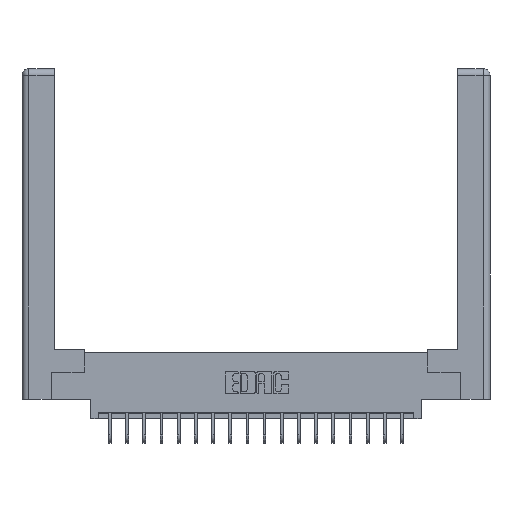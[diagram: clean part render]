
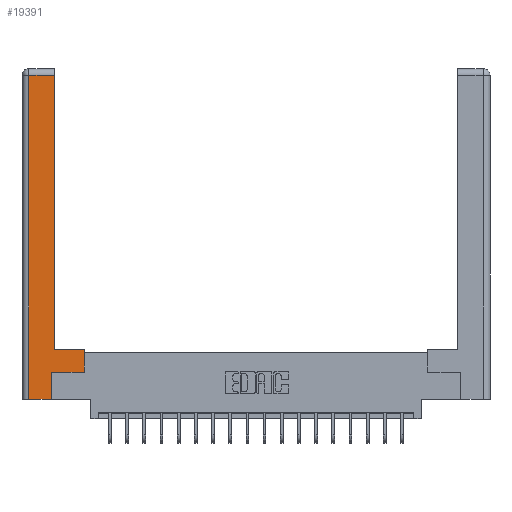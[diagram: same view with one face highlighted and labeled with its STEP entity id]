
A CAD part, top view. The second image highlights one B-rep face of the part: STEP entity #19391.
In plain terms, the highlighted planar face has unit normal (0, 0, 1).
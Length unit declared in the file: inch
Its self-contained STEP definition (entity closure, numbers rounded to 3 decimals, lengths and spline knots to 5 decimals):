
#118 = CARTESIAN_POINT ( 'NONE',  ( 0.0615, 2.94, 0. ) ) ;
#218 = EDGE_CURVE ( 'NONE', #1496, #2828, #5451, .T. ) ;
#439 = CARTESIAN_POINT ( 'NONE',  ( 0., 0., 0. ) ) ;
#492 = VERTEX_POINT ( 'NONE', #16414 ) ;
#513 = DIRECTION ( 'NONE',  ( 0., 0., -1. ) ) ;
#1148 = EDGE_CURVE ( 'NONE', #18475, #14431, #9116, .T. ) ;
#1348 = ORIENTED_EDGE ( 'NONE', *, *, #15074, .T. ) ;
#1496 = VERTEX_POINT ( 'NONE', #14817 ) ;
#1846 = ORIENTED_EDGE ( 'NONE', *, *, #1148, .T. ) ;
#1905 = DIRECTION ( 'NONE',  ( 1., 0., 0. ) ) ;
#2019 = LINE ( 'NONE', #16198, #3068 ) ;
#2564 = LINE ( 'NONE', #7671, #9888 ) ;
#2828 = VERTEX_POINT ( 'NONE', #8231 ) ;
#2836 = DIRECTION ( 'NONE',  ( 1., 0., 0. ) ) ;
#2910 = LINE ( 'NONE', #10985, #11253 ) ;
#3068 = VECTOR ( 'NONE', #18000, 39.37008 ) ;
#3588 = VERTEX_POINT ( 'NONE', #10169 ) ;
#3602 = EDGE_CURVE ( 'NONE', #20914, #492, #14079, .T. ) ;
#4310 = EDGE_CURVE ( 'NONE', #2828, #6431, #2019, .T. ) ;
#4472 = ORIENTED_EDGE ( 'NONE', *, *, #4310, .T. ) ;
#5004 = CARTESIAN_POINT ( 'NONE',  ( 0.265, 0.245, 0. ) ) ;
#5451 = LINE ( 'NONE', #21159, #21376 ) ;
#5739 = EDGE_LOOP ( 'NONE', ( #10432, #1846, #15015, #20598, #4472, #1348, #7565, #18660 ) ) ;
#5994 = VECTOR ( 'NONE', #21435, 39.37008 ) ;
#6321 = CARTESIAN_POINT ( 'NONE',  ( 0.0615, 2.94, 0. ) ) ;
#6431 = VERTEX_POINT ( 'NONE', #5004 ) ;
#7305 = CARTESIAN_POINT ( 'NONE',  ( 0.295, 2.94, 0. ) ) ;
#7557 = DIRECTION ( 'NONE',  ( 0., 1., 0. ) ) ;
#7565 = ORIENTED_EDGE ( 'NONE', *, *, #3602, .T. ) ;
#7671 = CARTESIAN_POINT ( 'NONE',  ( 0.0615, 0., 0. ) ) ;
#7690 = CARTESIAN_POINT ( 'NONE',  ( 0.295, 3., 0. ) ) ;
#8171 = DIRECTION ( 'NONE',  ( 0., -1., 0. ) ) ;
#8231 = CARTESIAN_POINT ( 'NONE',  ( 0.265, 0., 0. ) ) ;
#8362 = CARTESIAN_POINT ( 'NONE',  ( 0.565, 0.45, 0. ) ) ;
#8806 = VECTOR ( 'NONE', #1905, 39.37008 ) ;
#9116 = LINE ( 'NONE', #6321, #5994 ) ;
#9612 = VECTOR ( 'NONE', #7557, 39.37008 ) ;
#9888 = VECTOR ( 'NONE', #8171, 39.37008 ) ;
#9985 = EDGE_CURVE ( 'NONE', #492, #3588, #2910, .T. ) ;
#10169 = CARTESIAN_POINT ( 'NONE',  ( 0.295, 0.45, 0. ) ) ;
#10432 = ORIENTED_EDGE ( 'NONE', *, *, #17953, .T. ) ;
#10985 = CARTESIAN_POINT ( 'NONE',  ( 0.295, 0.45, 0. ) ) ;
#11115 = LINE ( 'NONE', #15179, #8806 ) ;
#11253 = VECTOR ( 'NONE', #15888, 39.37008 ) ;
#13243 = LINE ( 'NONE', #7690, #9612 ) ;
#13771 = PLANE ( 'NONE',  #18057 ) ;
#14079 = LINE ( 'NONE', #8362, #14336 ) ;
#14232 = EDGE_CURVE ( 'NONE', #14431, #1496, #2564, .T. ) ;
#14336 = VECTOR ( 'NONE', #20223, 39.37008 ) ;
#14431 = VERTEX_POINT ( 'NONE', #118 ) ;
#14473 = FACE_OUTER_BOUND ( 'NONE', #5739, .T. ) ;
#14817 = CARTESIAN_POINT ( 'NONE',  ( 0.0615, 0., 0. ) ) ;
#15015 = ORIENTED_EDGE ( 'NONE', *, *, #14232, .T. ) ;
#15074 = EDGE_CURVE ( 'NONE', #6431, #20914, #11115, .T. ) ;
#15179 = CARTESIAN_POINT ( 'NONE',  ( 0.565, 0.245, 0. ) ) ;
#15888 = DIRECTION ( 'NONE',  ( -1., 0., 0. ) ) ;
#16198 = CARTESIAN_POINT ( 'NONE',  ( 0.265, 0.245, 0. ) ) ;
#16414 = CARTESIAN_POINT ( 'NONE',  ( 0.565, 0.45, 0. ) ) ;
#17953 = EDGE_CURVE ( 'NONE', #3588, #18475, #13243, .T. ) ;
#18000 = DIRECTION ( 'NONE',  ( 0., 1., 0. ) ) ;
#18057 = AXIS2_PLACEMENT_3D ( 'NONE', #439, #513, #18582 ) ;
#18475 = VERTEX_POINT ( 'NONE', #7305 ) ;
#18582 = DIRECTION ( 'NONE',  ( -1., 0., 0. ) ) ;
#18660 = ORIENTED_EDGE ( 'NONE', *, *, #9985, .T. ) ;
#19391 = ADVANCED_FACE ( 'NONE', ( #14473 ), #13771, .F. ) ;
#20223 = DIRECTION ( 'NONE',  ( 0., 1., 0. ) ) ;
#20598 = ORIENTED_EDGE ( 'NONE', *, *, #218, .T. ) ;
#20914 = VERTEX_POINT ( 'NONE', #21517 ) ;
#21159 = CARTESIAN_POINT ( 'NONE',  ( 0.265, 0., 0. ) ) ;
#21376 = VECTOR ( 'NONE', #2836, 39.37008 ) ;
#21435 = DIRECTION ( 'NONE',  ( -1., 0., 0. ) ) ;
#21517 = CARTESIAN_POINT ( 'NONE',  ( 0.565, 0.245, 0. ) ) ;
